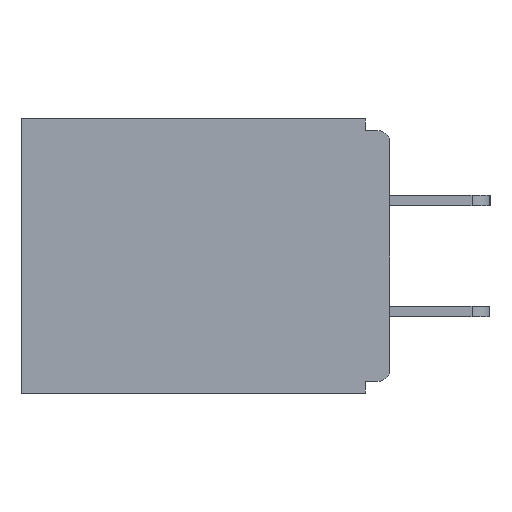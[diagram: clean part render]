
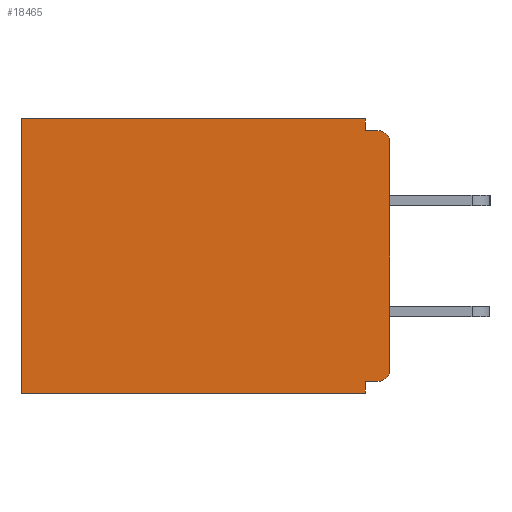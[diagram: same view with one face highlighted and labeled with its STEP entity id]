
A CAD part, left-side view. The second image highlights one B-rep face of the part: STEP entity #18465.
In plain terms, the highlighted planar face has unit normal (-1, 0, 0).
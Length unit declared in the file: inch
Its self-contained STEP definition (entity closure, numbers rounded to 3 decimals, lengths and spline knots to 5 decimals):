
#77 = AXIS2_PLACEMENT_3D ( 'NONE', #407, #10766, #12563 ) ;
#111 = ORIENTED_EDGE ( 'NONE', *, *, #17604, .F. ) ;
#262 = ORIENTED_EDGE ( 'NONE', *, *, #9059, .F. ) ;
#407 = CARTESIAN_POINT ( 'NONE',  ( 0.298, 0.015, -0.313 ) ) ;
#585 = VERTEX_POINT ( 'NONE', #14917 ) ;
#754 = ORIENTED_EDGE ( 'NONE', *, *, #19453, .T. ) ;
#833 = DIRECTION ( 'NONE',  ( 0., 0., -1. ) ) ;
#1066 = VERTEX_POINT ( 'NONE', #19573 ) ;
#1146 = ORIENTED_EDGE ( 'NONE', *, *, #1563, .F. ) ;
#1563 = EDGE_CURVE ( 'NONE', #19707, #16346, #15622, .T. ) ;
#1806 = CARTESIAN_POINT ( 'NONE',  ( 0.298, 0., 0. ) ) ;
#2035 = DIRECTION ( 'NONE',  ( 0., 1., 0. ) ) ;
#2217 = CARTESIAN_POINT ( 'NONE',  ( 0.298, 0., 0. ) ) ;
#2599 = VERTEX_POINT ( 'NONE', #3961 ) ;
#2605 = EDGE_LOOP ( 'NONE', ( #754, #16384, #14158, #6704, #4132, #13845, #262, #111, #8448, #1146 ) ) ;
#3652 = PLANE ( 'NONE',  #15647 ) ;
#3902 = LINE ( 'NONE', #11725, #12982 ) ;
#3961 = CARTESIAN_POINT ( 'NONE',  ( 0.298, 0.46, -0.343 ) ) ;
#4132 = ORIENTED_EDGE ( 'NONE', *, *, #4681, .T. ) ;
#4265 = DIRECTION ( 'NONE',  ( -1., 0., 0. ) ) ;
#4681 = EDGE_CURVE ( 'NONE', #13871, #2599, #5446, .T. ) ;
#4683 = LINE ( 'NONE', #18562, #13734 ) ;
#4867 = DIRECTION ( 'NONE',  ( 0., -1., 0. ) ) ;
#5049 = CARTESIAN_POINT ( 'NONE',  ( 0.298, 0.015, -0.03 ) ) ;
#5308 = CARTESIAN_POINT ( 'NONE',  ( 0.298, 0.46, 0. ) ) ;
#5446 = LINE ( 'NONE', #6152, #9400 ) ;
#5765 = DIRECTION ( 'NONE',  ( 0., 0., -1. ) ) ;
#6152 = CARTESIAN_POINT ( 'NONE',  ( 0.298, 0.46, 0. ) ) ;
#6166 = EDGE_CURVE ( 'NONE', #14260, #13871, #11597, .T. ) ;
#6663 = DIRECTION ( 'NONE',  ( 0., 1., 0. ) ) ;
#6704 = ORIENTED_EDGE ( 'NONE', *, *, #6166, .T. ) ;
#6964 = EDGE_CURVE ( 'NONE', #7159, #16346, #10478, .T. ) ;
#6967 = DIRECTION ( 'NONE',  ( 1., 0., 0. ) ) ;
#7109 = DIRECTION ( 'NONE',  ( 0., 0., -1. ) ) ;
#7159 = VERTEX_POINT ( 'NONE', #9766 ) ;
#7441 = CARTESIAN_POINT ( 'NONE',  ( 0.298, 0.031, 0. ) ) ;
#7946 = AXIS2_PLACEMENT_3D ( 'NONE', #5049, #4265, #8355 ) ;
#7957 = CARTESIAN_POINT ( 'NONE',  ( 0.298, 0., -0.313 ) ) ;
#8164 = FACE_OUTER_BOUND ( 'NONE', #2605, .T. ) ;
#8355 = DIRECTION ( 'NONE',  ( 0., 0., -1. ) ) ;
#8448 = ORIENTED_EDGE ( 'NONE', *, *, #6964, .T. ) ;
#8752 = EDGE_CURVE ( 'NONE', #14260, #15136, #13620, .T. ) ;
#9051 = LINE ( 'NONE', #11428, #16482 ) ;
#9059 = EDGE_CURVE ( 'NONE', #585, #1066, #9051, .T. ) ;
#9400 = VECTOR ( 'NONE', #833, 39.37008 ) ;
#9766 = CARTESIAN_POINT ( 'NONE',  ( 0.298, 0.015, -0.328 ) ) ;
#10343 = CARTESIAN_POINT ( 'NONE',  ( 0.298, 0.031, -0.015 ) ) ;
#10478 = CIRCLE ( 'NONE', #77, 0.015 ) ;
#10766 = DIRECTION ( 'NONE',  ( -1., 0., 0. ) ) ;
#11428 = CARTESIAN_POINT ( 'NONE',  ( 0.298, 0.031, -0.343 ) ) ;
#11512 = VECTOR ( 'NONE', #14904, 39.37008 ) ;
#11597 = LINE ( 'NONE', #14114, #12648 ) ;
#11725 = CARTESIAN_POINT ( 'NONE',  ( 0.298, 0., -0.343 ) ) ;
#12532 = LINE ( 'NONE', #20060, #16455 ) ;
#12563 = DIRECTION ( 'NONE',  ( 0., 0., -1. ) ) ;
#12648 = VECTOR ( 'NONE', #2035, 39.37008 ) ;
#12982 = VECTOR ( 'NONE', #18407, 39.37008 ) ;
#13117 = DIRECTION ( 'NONE',  ( 0., 0., -1. ) ) ;
#13220 = CARTESIAN_POINT ( 'NONE',  ( 0.298, 0.031, -0.343 ) ) ;
#13620 = LINE ( 'NONE', #13220, #11512 ) ;
#13734 = VECTOR ( 'NONE', #6663, 39.37008 ) ;
#13845 = ORIENTED_EDGE ( 'NONE', *, *, #17147, .F. ) ;
#13871 = VERTEX_POINT ( 'NONE', #5308 ) ;
#14114 = CARTESIAN_POINT ( 'NONE',  ( 0.298, 0., 0. ) ) ;
#14158 = ORIENTED_EDGE ( 'NONE', *, *, #8752, .F. ) ;
#14260 = VERTEX_POINT ( 'NONE', #7441 ) ;
#14652 = CARTESIAN_POINT ( 'NONE',  ( 0.298, 0., -0.03 ) ) ;
#14904 = DIRECTION ( 'NONE',  ( 0., 0., -1. ) ) ;
#14917 = CARTESIAN_POINT ( 'NONE',  ( 0.298, 0.031, -0.328 ) ) ;
#15136 = VERTEX_POINT ( 'NONE', #10343 ) ;
#15622 = LINE ( 'NONE', #2217, #19034 ) ;
#15647 = AXIS2_PLACEMENT_3D ( 'NONE', #1806, #6967, #7109 ) ;
#15806 = EDGE_CURVE ( 'NONE', #15136, #21964, #12532, .T. ) ;
#16346 = VERTEX_POINT ( 'NONE', #7957 ) ;
#16384 = ORIENTED_EDGE ( 'NONE', *, *, #15806, .F. ) ;
#16455 = VECTOR ( 'NONE', #4867, 39.37008 ) ;
#16482 = VECTOR ( 'NONE', #13117, 39.37008 ) ;
#17147 = EDGE_CURVE ( 'NONE', #1066, #2599, #3902, .T. ) ;
#17604 = EDGE_CURVE ( 'NONE', #7159, #585, #4683, .T. ) ;
#17649 = CARTESIAN_POINT ( 'NONE',  ( 0.298, 0.015, -0.015 ) ) ;
#18407 = DIRECTION ( 'NONE',  ( 0., 1., 0. ) ) ;
#18465 = ADVANCED_FACE ( 'NONE', ( #8164 ), #3652, .F. ) ;
#18562 = CARTESIAN_POINT ( 'NONE',  ( 0.298, 0., -0.328 ) ) ;
#19034 = VECTOR ( 'NONE', #5765, 39.37008 ) ;
#19453 = EDGE_CURVE ( 'NONE', #19707, #21964, #21138, .T. ) ;
#19573 = CARTESIAN_POINT ( 'NONE',  ( 0.298, 0.031, -0.343 ) ) ;
#19707 = VERTEX_POINT ( 'NONE', #14652 ) ;
#20060 = CARTESIAN_POINT ( 'NONE',  ( 0.298, 0., -0.015 ) ) ;
#21138 = CIRCLE ( 'NONE', #7946, 0.015 ) ;
#21964 = VERTEX_POINT ( 'NONE', #17649 ) ;
